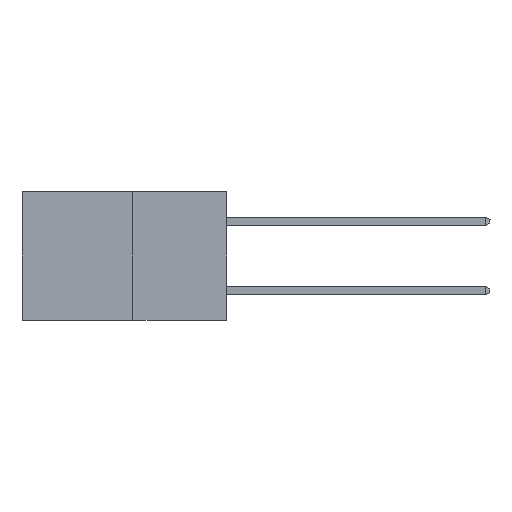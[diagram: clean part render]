
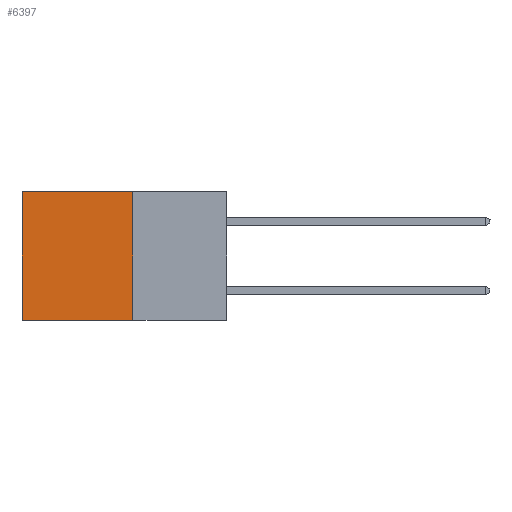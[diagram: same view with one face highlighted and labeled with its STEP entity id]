
A CAD part, left-side view. The second image highlights one B-rep face of the part: STEP entity #6397.
In plain terms, the highlighted planar face has unit normal (-1, 0, 0).
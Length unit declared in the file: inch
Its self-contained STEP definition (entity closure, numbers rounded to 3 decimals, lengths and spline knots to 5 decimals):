
#212 = VECTOR ( 'NONE', #16724, 39.37008 ) ;
#473 = ORIENTED_EDGE ( 'NONE', *, *, #485, .T. ) ;
#485 = EDGE_CURVE ( 'NONE', #11811, #6620, #18679, .T. ) ;
#1321 = CARTESIAN_POINT ( 'NONE',  ( 0.277, 0.27, 0. ) ) ;
#2303 = ORIENTED_EDGE ( 'NONE', *, *, #12192, .F. ) ;
#2376 = VECTOR ( 'NONE', #18734, 39.37008 ) ;
#2448 = VECTOR ( 'NONE', #2674, 39.37008 ) ;
#2674 = DIRECTION ( 'NONE',  ( 0., 0., -1. ) ) ;
#4593 = DIRECTION ( 'NONE',  ( 0., 0., -1. ) ) ;
#4614 = VECTOR ( 'NONE', #4593, 39.37008 ) ;
#5096 = CARTESIAN_POINT ( 'NONE',  ( 0.277, 0.27, 0. ) ) ;
#6397 = ADVANCED_FACE ( 'NONE', ( #12635 ), #18097, .F. ) ;
#6620 = VERTEX_POINT ( 'NONE', #14134 ) ;
#6798 = CARTESIAN_POINT ( 'NONE',  ( 0.277, 0.59, -0.37 ) ) ;
#8032 = DIRECTION ( 'NONE',  ( 0., 0., -1. ) ) ;
#8098 = CARTESIAN_POINT ( 'NONE',  ( 0.277, 0.27, -0.37 ) ) ;
#8755 = EDGE_CURVE ( 'NONE', #12478, #14778, #8880, .T. ) ;
#8880 = LINE ( 'NONE', #13528, #4614 ) ;
#9787 = ORIENTED_EDGE ( 'NONE', *, *, #9844, .T. ) ;
#9844 = EDGE_CURVE ( 'NONE', #12478, #11811, #12746, .T. ) ;
#10863 = CARTESIAN_POINT ( 'NONE',  ( 0.277, 0.59, 0. ) ) ;
#11104 = ORIENTED_EDGE ( 'NONE', *, *, #8755, .F. ) ;
#11811 = VERTEX_POINT ( 'NONE', #10863 ) ;
#12192 = EDGE_CURVE ( 'NONE', #14778, #6620, #15158, .T. ) ;
#12442 = DIRECTION ( 'NONE',  ( 1., 0., 0. ) ) ;
#12478 = VERTEX_POINT ( 'NONE', #1321 ) ;
#12509 = CARTESIAN_POINT ( 'NONE',  ( 0.277, 0.27, -0.37 ) ) ;
#12635 = FACE_OUTER_BOUND ( 'NONE', #14562, .T. ) ;
#12746 = LINE ( 'NONE', #5096, #212 ) ;
#13528 = CARTESIAN_POINT ( 'NONE',  ( 0.277, 0.27, -0.37 ) ) ;
#14134 = CARTESIAN_POINT ( 'NONE',  ( 0.277, 0.59, -0.37 ) ) ;
#14562 = EDGE_LOOP ( 'NONE', ( #473, #2303, #11104, #9787 ) ) ;
#14778 = VERTEX_POINT ( 'NONE', #8098 ) ;
#15158 = LINE ( 'NONE', #18919, #2376 ) ;
#16724 = DIRECTION ( 'NONE',  ( 0., 1., 0. ) ) ;
#17827 = AXIS2_PLACEMENT_3D ( 'NONE', #12509, #12442, #8032 ) ;
#18097 = PLANE ( 'NONE',  #17827 ) ;
#18679 = LINE ( 'NONE', #6798, #2448 ) ;
#18734 = DIRECTION ( 'NONE',  ( 0., 1., 0. ) ) ;
#18919 = CARTESIAN_POINT ( 'NONE',  ( 0.277, 0.27, -0.37 ) ) ;
